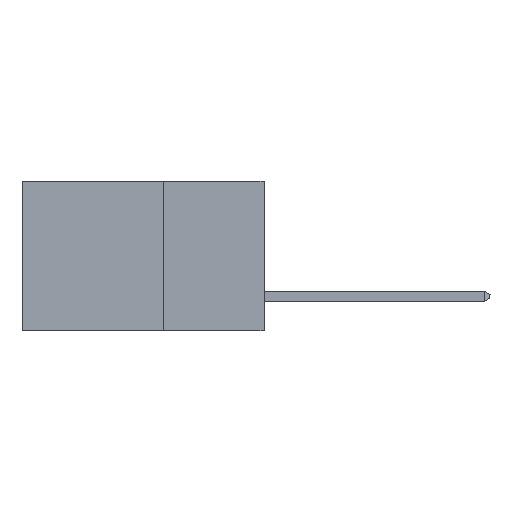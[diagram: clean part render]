
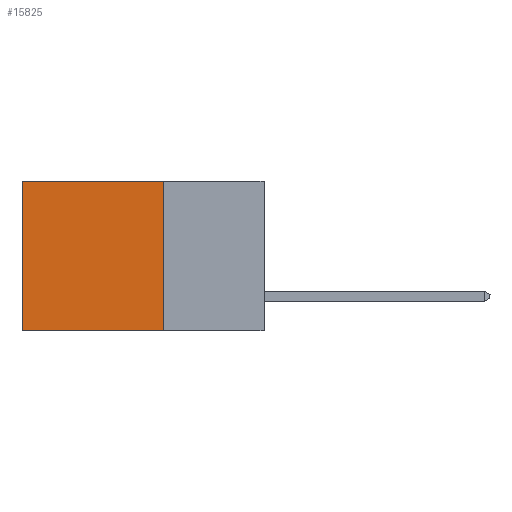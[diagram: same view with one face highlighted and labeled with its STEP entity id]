
A CAD part, left-side view. The second image highlights one B-rep face of the part: STEP entity #15825.
In plain terms, the highlighted planar face has unit normal (-1, 0, 0).
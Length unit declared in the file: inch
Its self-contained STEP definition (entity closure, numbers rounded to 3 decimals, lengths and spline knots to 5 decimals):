
#17 = EDGE_CURVE ( 'NONE', #21299, #1756, #2592, .T. ) ;
#423 = DIRECTION ( 'NONE',  ( 0., 1., 0. ) ) ;
#981 = LINE ( 'NONE', #1106, #11550 ) ;
#1106 = CARTESIAN_POINT ( 'NONE',  ( 0.2615, 0.25, -0.37 ) ) ;
#1669 = DIRECTION ( 'NONE',  ( 0., 0., -1. ) ) ;
#1756 = VERTEX_POINT ( 'NONE', #10912 ) ;
#2148 = VERTEX_POINT ( 'NONE', #6140 ) ;
#2287 = VECTOR ( 'NONE', #14037, 39.37008 ) ;
#2592 = LINE ( 'NONE', #4175, #11641 ) ;
#3397 = DIRECTION ( 'NONE',  ( 0., 0., -1. ) ) ;
#4175 = CARTESIAN_POINT ( 'NONE',  ( 0.2615, 0.25, -0.37 ) ) ;
#5551 = FACE_OUTER_BOUND ( 'NONE', #10768, .T. ) ;
#6140 = CARTESIAN_POINT ( 'NONE',  ( 0.2615, 0.25, 0. ) ) ;
#6230 = EDGE_CURVE ( 'NONE', #2148, #10883, #22082, .T. ) ;
#7998 = CARTESIAN_POINT ( 'NONE',  ( 0.2615, 0.6, 0. ) ) ;
#10190 = LINE ( 'NONE', #17857, #2287 ) ;
#10768 = EDGE_LOOP ( 'NONE', ( #21977, #13582, #19975, #11668 ) ) ;
#10883 = VERTEX_POINT ( 'NONE', #7998 ) ;
#10912 = CARTESIAN_POINT ( 'NONE',  ( 0.2615, 0.6, -0.37 ) ) ;
#11550 = VECTOR ( 'NONE', #1669, 39.37008 ) ;
#11641 = VECTOR ( 'NONE', #423, 39.37008 ) ;
#11668 = ORIENTED_EDGE ( 'NONE', *, *, #6230, .T. ) ;
#12672 = VECTOR ( 'NONE', #20740, 39.37008 ) ;
#13508 = EDGE_CURVE ( 'NONE', #10883, #1756, #10190, .T. ) ;
#13582 = ORIENTED_EDGE ( 'NONE', *, *, #17, .F. ) ;
#14037 = DIRECTION ( 'NONE',  ( 0., 0., -1. ) ) ;
#14405 = EDGE_CURVE ( 'NONE', #2148, #21299, #981, .T. ) ;
#14594 = CARTESIAN_POINT ( 'NONE',  ( 0.2615, 0.25, -0.37 ) ) ;
#14819 = DIRECTION ( 'NONE',  ( 1., 0., 0. ) ) ;
#15825 = ADVANCED_FACE ( 'NONE', ( #5551 ), #18053, .F. ) ;
#16780 = CARTESIAN_POINT ( 'NONE',  ( 0.2615, 0.25, -0.37 ) ) ;
#16900 = CARTESIAN_POINT ( 'NONE',  ( 0.2615, 0.25, 0. ) ) ;
#17857 = CARTESIAN_POINT ( 'NONE',  ( 0.2615, 0.6, -0.37 ) ) ;
#18053 = PLANE ( 'NONE',  #18873 ) ;
#18873 = AXIS2_PLACEMENT_3D ( 'NONE', #14594, #14819, #3397 ) ;
#19975 = ORIENTED_EDGE ( 'NONE', *, *, #14405, .F. ) ;
#20740 = DIRECTION ( 'NONE',  ( 0., 1., 0. ) ) ;
#21299 = VERTEX_POINT ( 'NONE', #16780 ) ;
#21977 = ORIENTED_EDGE ( 'NONE', *, *, #13508, .T. ) ;
#22082 = LINE ( 'NONE', #16900, #12672 ) ;
